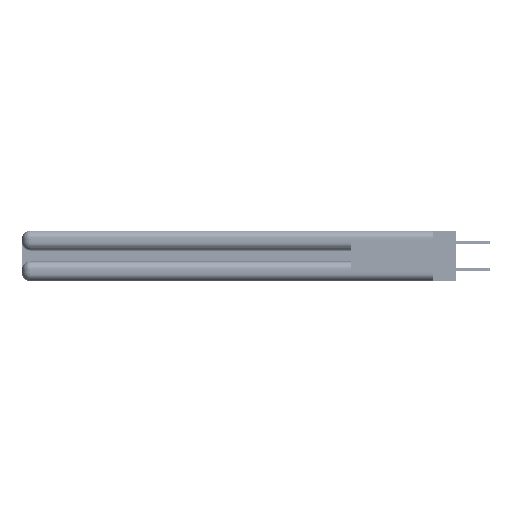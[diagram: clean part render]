
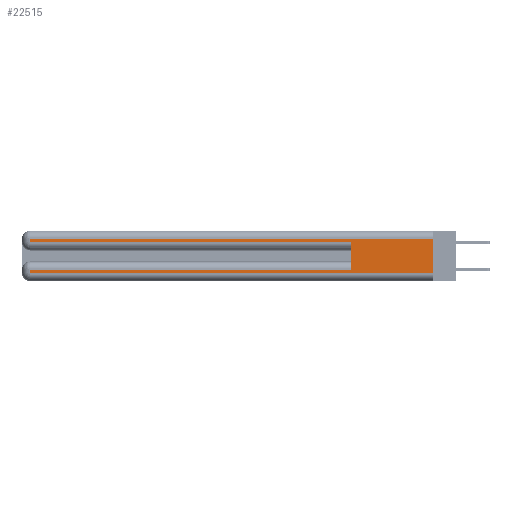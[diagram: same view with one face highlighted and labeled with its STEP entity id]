
A CAD part, left-side view. The second image highlights one B-rep face of the part: STEP entity #22515.
In plain terms, the highlighted planar face has unit normal (-1, 0, 0).
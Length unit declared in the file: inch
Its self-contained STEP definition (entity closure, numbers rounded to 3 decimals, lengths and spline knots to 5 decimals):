
#3659 = ORIENTED_EDGE ( 'NONE', *, *, #18998, .F. ) ;
#4312 = VECTOR ( 'NONE', #28347, 39.37008 ) ;
#4557 = CARTESIAN_POINT ( 'NONE',  ( 0., 0., 0.31 ) ) ;
#6713 = VERTEX_POINT ( 'NONE', #13619 ) ;
#6773 = LINE ( 'NONE', #22717, #7998 ) ;
#7434 = CARTESIAN_POINT ( 'NONE',  ( 0., 0., 0.06 ) ) ;
#7998 = VECTOR ( 'NONE', #11261, 39.37008 ) ;
#8325 = CARTESIAN_POINT ( 'NONE',  ( 0., 2.94, 0.37 ) ) ;
#10216 = VECTOR ( 'NONE', #30989, 39.37008 ) ;
#11261 = DIRECTION ( 'NONE',  ( 0., 0., 1. ) ) ;
#12723 = VECTOR ( 'NONE', #16734, 39.37008 ) ;
#13619 = CARTESIAN_POINT ( 'NONE',  ( 0., 0., 0.06 ) ) ;
#14086 = LINE ( 'NONE', #44039, #4312 ) ;
#16492 = LINE ( 'NONE', #21150, #46999 ) ;
#16734 = DIRECTION ( 'NONE',  ( 0., 0., -1. ) ) ;
#17202 = LINE ( 'NONE', #48203, #44671 ) ;
#17477 = DIRECTION ( 'NONE',  ( 0., 0., -1. ) ) ;
#18029 = ORIENTED_EDGE ( 'NONE', *, *, #48435, .T. ) ;
#18998 = EDGE_CURVE ( 'NONE', #24058, #31639, #6773, .T. ) ;
#19859 = LINE ( 'NONE', #48434, #40592 ) ;
#20614 = LINE ( 'NONE', #7434, #10216 ) ;
#21150 = CARTESIAN_POINT ( 'NONE',  ( 0., 0., 0.085 ) ) ;
#22515 = ADVANCED_FACE ( 'NONE', ( #48068 ), #49071, .F. ) ;
#22717 = CARTESIAN_POINT ( 'NONE',  ( 0., 0.6, 0.145 ) ) ;
#22721 = CARTESIAN_POINT ( 'NONE',  ( 0., 2.94, 0.31 ) ) ;
#23428 = CARTESIAN_POINT ( 'NONE',  ( 0., 2.94, 0.085 ) ) ;
#23669 = EDGE_CURVE ( 'NONE', #29110, #43099, #19859, .T. ) ;
#24058 = VERTEX_POINT ( 'NONE', #32032 ) ;
#25401 = DIRECTION ( 'NONE',  ( 0., 1., 0. ) ) ;
#25522 = EDGE_CURVE ( 'NONE', #43099, #34142, #17202, .T. ) ;
#25679 = CARTESIAN_POINT ( 'NONE',  ( 0., 0., 0.37 ) ) ;
#26022 = EDGE_CURVE ( 'NONE', #34142, #31639, #14086, .T. ) ;
#26771 = EDGE_CURVE ( 'NONE', #28008, #46701, #28587, .T. ) ;
#27229 = EDGE_CURVE ( 'NONE', #46701, #6713, #20614, .T. ) ;
#28008 = VERTEX_POINT ( 'NONE', #23428 ) ;
#28347 = DIRECTION ( 'NONE',  ( 0., -1., 0. ) ) ;
#28587 = LINE ( 'NONE', #8325, #12723 ) ;
#29075 = DIRECTION ( 'NONE',  ( 0., 0., -1. ) ) ;
#29110 = VERTEX_POINT ( 'NONE', #4557 ) ;
#29605 = DIRECTION ( 'NONE',  ( 0., 0., -1. ) ) ;
#30989 = DIRECTION ( 'NONE',  ( 0., -1., 0. ) ) ;
#31639 = VERTEX_POINT ( 'NONE', #35211 ) ;
#32032 = CARTESIAN_POINT ( 'NONE',  ( 0., 0.6, 0.085 ) ) ;
#32360 = ORIENTED_EDGE ( 'NONE', *, *, #38808, .F. ) ;
#33110 = DIRECTION ( 'NONE',  ( 0., 1., 0. ) ) ;
#34142 = VERTEX_POINT ( 'NONE', #38379 ) ;
#35211 = CARTESIAN_POINT ( 'NONE',  ( 0., 0.6, 0.285 ) ) ;
#37095 = CARTESIAN_POINT ( 'NONE',  ( 0., 0., 0.37 ) ) ;
#37232 = LINE ( 'NONE', #37095, #46394 ) ;
#38379 = CARTESIAN_POINT ( 'NONE',  ( 0., 2.94, 0.285 ) ) ;
#38808 = EDGE_CURVE ( 'NONE', #29110, #6713, #37232, .T. ) ;
#38850 = ORIENTED_EDGE ( 'NONE', *, *, #25522, .T. ) ;
#40592 = VECTOR ( 'NONE', #25401, 39.37008 ) ;
#41532 = DIRECTION ( 'NONE',  ( 1., 0., 0. ) ) ;
#43097 = ORIENTED_EDGE ( 'NONE', *, *, #23669, .T. ) ;
#43099 = VERTEX_POINT ( 'NONE', #22721 ) ;
#44039 = CARTESIAN_POINT ( 'NONE',  ( 0., 0., 0.285 ) ) ;
#44671 = VECTOR ( 'NONE', #29075, 39.37008 ) ;
#44950 = AXIS2_PLACEMENT_3D ( 'NONE', #25679, #41532, #29605 ) ;
#46147 = EDGE_LOOP ( 'NONE', ( #32360, #43097, #38850, #48605, #3659, #18029, #48059, #46818 ) ) ;
#46394 = VECTOR ( 'NONE', #17477, 39.37008 ) ;
#46651 = CARTESIAN_POINT ( 'NONE',  ( 0., 2.94, 0.06 ) ) ;
#46701 = VERTEX_POINT ( 'NONE', #46651 ) ;
#46818 = ORIENTED_EDGE ( 'NONE', *, *, #27229, .T. ) ;
#46999 = VECTOR ( 'NONE', #33110, 39.37008 ) ;
#48059 = ORIENTED_EDGE ( 'NONE', *, *, #26771, .T. ) ;
#48068 = FACE_OUTER_BOUND ( 'NONE', #46147, .T. ) ;
#48203 = CARTESIAN_POINT ( 'NONE',  ( 0., 2.94, 0.37 ) ) ;
#48434 = CARTESIAN_POINT ( 'NONE',  ( 0., 0., 0.31 ) ) ;
#48435 = EDGE_CURVE ( 'NONE', #24058, #28008, #16492, .T. ) ;
#48605 = ORIENTED_EDGE ( 'NONE', *, *, #26022, .T. ) ;
#49071 = PLANE ( 'NONE',  #44950 ) ;
